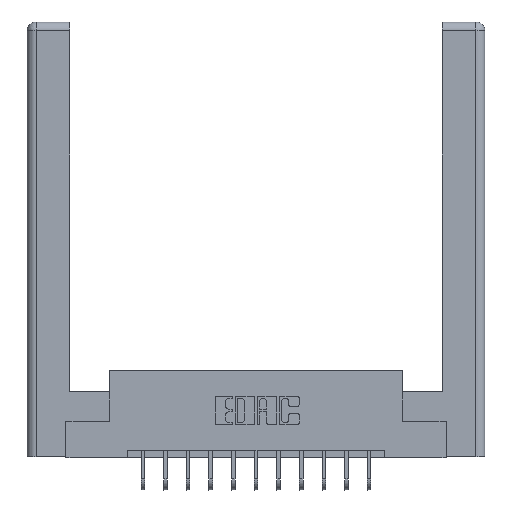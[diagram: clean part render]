
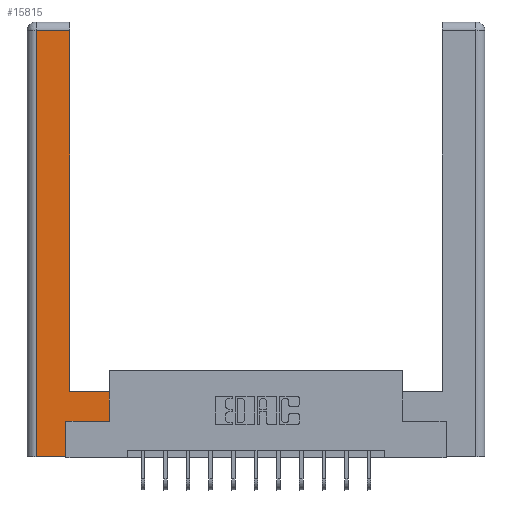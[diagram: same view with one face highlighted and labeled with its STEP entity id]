
A CAD part, top view. The second image highlights one B-rep face of the part: STEP entity #15815.
In plain terms, the highlighted planar face has unit normal (0, 0, 1).
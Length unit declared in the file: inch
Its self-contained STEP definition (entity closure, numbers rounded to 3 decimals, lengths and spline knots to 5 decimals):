
#6 = CARTESIAN_POINT ( 'NONE',  ( 0.565, 0.245, 0. ) ) ;
#278 = CARTESIAN_POINT ( 'NONE',  ( 0.295, 3., 0. ) ) ;
#359 = DIRECTION ( 'NONE',  ( 0., -1., 0. ) ) ;
#620 = DIRECTION ( 'NONE',  ( 0., 0., -1. ) ) ;
#988 = CARTESIAN_POINT ( 'NONE',  ( 0.0615, 0., 0. ) ) ;
#1242 = AXIS2_PLACEMENT_3D ( 'NONE', #11060, #620, #16310 ) ;
#1268 = VECTOR ( 'NONE', #359, 39.37008 ) ;
#1639 = CARTESIAN_POINT ( 'NONE',  ( 0.0615, 2.94, 0. ) ) ;
#2072 = ORIENTED_EDGE ( 'NONE', *, *, #7417, .T. ) ;
#2257 = CARTESIAN_POINT ( 'NONE',  ( 0.0615, 2.94, 0. ) ) ;
#2790 = EDGE_CURVE ( 'NONE', #8754, #10508, #15295, .T. ) ;
#3088 = CARTESIAN_POINT ( 'NONE',  ( 0.0615, 0., 0. ) ) ;
#3118 = EDGE_CURVE ( 'NONE', #14581, #8806, #3959, .T. ) ;
#3896 = EDGE_CURVE ( 'NONE', #7934, #14581, #6170, .T. ) ;
#3959 = LINE ( 'NONE', #1639, #13431 ) ;
#4324 = LINE ( 'NONE', #3088, #1268 ) ;
#4736 = ORIENTED_EDGE ( 'NONE', *, *, #3896, .T. ) ;
#4758 = FACE_OUTER_BOUND ( 'NONE', #14647, .T. ) ;
#5058 = VECTOR ( 'NONE', #13307, 39.37008 ) ;
#5797 = VERTEX_POINT ( 'NONE', #11973 ) ;
#6115 = VECTOR ( 'NONE', #13127, 39.37008 ) ;
#6170 = LINE ( 'NONE', #278, #7200 ) ;
#6332 = DIRECTION ( 'NONE',  ( 1., 0., 0. ) ) ;
#6663 = LINE ( 'NONE', #14854, #10727 ) ;
#6680 = VECTOR ( 'NONE', #14550, 39.37008 ) ;
#7200 = VECTOR ( 'NONE', #10755, 39.37008 ) ;
#7346 = LINE ( 'NONE', #9245, #6115 ) ;
#7398 = CARTESIAN_POINT ( 'NONE',  ( 0.265, 0., 0. ) ) ;
#7417 = EDGE_CURVE ( 'NONE', #10508, #16663, #15942, .T. ) ;
#7434 = CARTESIAN_POINT ( 'NONE',  ( 0.295, 2.94, 0. ) ) ;
#7934 = VERTEX_POINT ( 'NONE', #11443 ) ;
#8477 = DIRECTION ( 'NONE',  ( 0., 1., 0. ) ) ;
#8754 = VERTEX_POINT ( 'NONE', #988 ) ;
#8784 = EDGE_CURVE ( 'NONE', #16663, #12867, #15074, .T. ) ;
#8806 = VERTEX_POINT ( 'NONE', #2257 ) ;
#9245 = CARTESIAN_POINT ( 'NONE',  ( 0.295, 0.45, 0. ) ) ;
#9358 = ORIENTED_EDGE ( 'NONE', *, *, #8784, .T. ) ;
#9429 = CARTESIAN_POINT ( 'NONE',  ( 0.265, 0.245, 0. ) ) ;
#9820 = CARTESIAN_POINT ( 'NONE',  ( 0.265, 0., 0. ) ) ;
#10017 = CARTESIAN_POINT ( 'NONE',  ( 0.565, 0.245, 0. ) ) ;
#10136 = VECTOR ( 'NONE', #6332, 39.37008 ) ;
#10168 = ORIENTED_EDGE ( 'NONE', *, *, #16315, .T. ) ;
#10187 = CARTESIAN_POINT ( 'NONE',  ( 0.265, 0.245, 0. ) ) ;
#10508 = VERTEX_POINT ( 'NONE', #9820 ) ;
#10681 = ORIENTED_EDGE ( 'NONE', *, *, #11700, .T. ) ;
#10727 = VECTOR ( 'NONE', #8477, 39.37008 ) ;
#10755 = DIRECTION ( 'NONE',  ( 0., 1., 0. ) ) ;
#11060 = CARTESIAN_POINT ( 'NONE',  ( 0., 0., 0. ) ) ;
#11443 = CARTESIAN_POINT ( 'NONE',  ( 0.295, 0.45, 0. ) ) ;
#11700 = EDGE_CURVE ( 'NONE', #5797, #7934, #7346, .T. ) ;
#11973 = CARTESIAN_POINT ( 'NONE',  ( 0.565, 0.45, 0. ) ) ;
#12276 = ORIENTED_EDGE ( 'NONE', *, *, #2790, .T. ) ;
#12483 = PLANE ( 'NONE',  #1242 ) ;
#12867 = VERTEX_POINT ( 'NONE', #6 ) ;
#13127 = DIRECTION ( 'NONE',  ( -1., 0., 0. ) ) ;
#13307 = DIRECTION ( 'NONE',  ( 0., 1., 0. ) ) ;
#13431 = VECTOR ( 'NONE', #14597, 39.37008 ) ;
#13619 = ORIENTED_EDGE ( 'NONE', *, *, #3118, .T. ) ;
#14550 = DIRECTION ( 'NONE',  ( 1., 0., 0. ) ) ;
#14581 = VERTEX_POINT ( 'NONE', #7434 ) ;
#14597 = DIRECTION ( 'NONE',  ( -1., 0., 0. ) ) ;
#14647 = EDGE_LOOP ( 'NONE', ( #4736, #13619, #10168, #12276, #2072, #9358, #16752, #10681 ) ) ;
#14854 = CARTESIAN_POINT ( 'NONE',  ( 0.565, 0.45, 0. ) ) ;
#15062 = EDGE_CURVE ( 'NONE', #12867, #5797, #6663, .T. ) ;
#15074 = LINE ( 'NONE', #10017, #10136 ) ;
#15295 = LINE ( 'NONE', #7398, #6680 ) ;
#15815 = ADVANCED_FACE ( 'NONE', ( #4758 ), #12483, .F. ) ;
#15942 = LINE ( 'NONE', #9429, #5058 ) ;
#16310 = DIRECTION ( 'NONE',  ( -1., 0., 0. ) ) ;
#16315 = EDGE_CURVE ( 'NONE', #8806, #8754, #4324, .T. ) ;
#16663 = VERTEX_POINT ( 'NONE', #10187 ) ;
#16752 = ORIENTED_EDGE ( 'NONE', *, *, #15062, .T. ) ;
